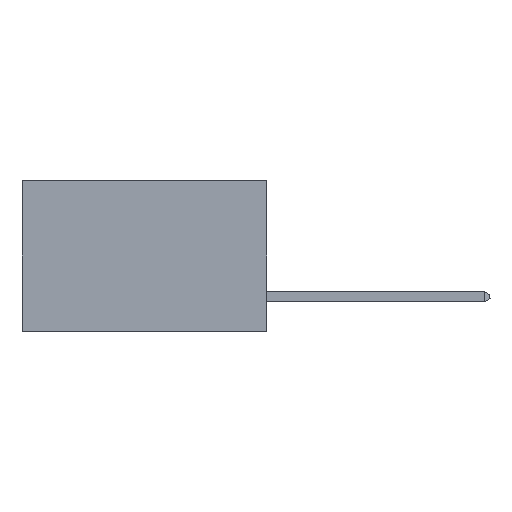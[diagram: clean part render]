
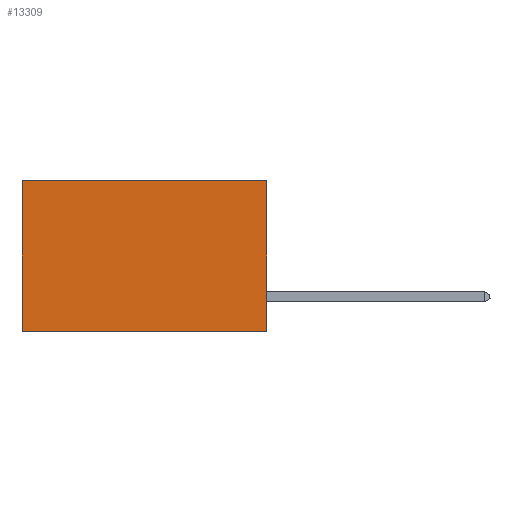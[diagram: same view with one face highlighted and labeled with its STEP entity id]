
A CAD part, left-side view. The second image highlights one B-rep face of the part: STEP entity #13309.
In plain terms, the highlighted planar face has unit normal (-1, 0, 0).
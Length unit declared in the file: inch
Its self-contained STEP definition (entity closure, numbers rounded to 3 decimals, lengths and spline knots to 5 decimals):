
#159 = AXIS2_PLACEMENT_3D ( 'NONE', #29523, #40713, #29852 ) ;
#1380 = ORIENTED_EDGE ( 'NONE', *, *, #31086, .F. ) ;
#3466 = PLANE ( 'NONE',  #159 ) ;
#7164 = EDGE_LOOP ( 'NONE', ( #7315, #12968, #1380, #22053 ) ) ;
#7315 = ORIENTED_EDGE ( 'NONE', *, *, #12239, .T. ) ;
#7946 = VERTEX_POINT ( 'NONE', #32042 ) ;
#8079 = CARTESIAN_POINT ( 'NONE',  ( 0.2875, 0.6, 0. ) ) ;
#8308 = CARTESIAN_POINT ( 'NONE',  ( 0.2875, 0., -0.37 ) ) ;
#10257 = EDGE_CURVE ( 'NONE', #40282, #7946, #44008, .T. ) ;
#11302 = CARTESIAN_POINT ( 'NONE',  ( 0.2875, 0., -0.37 ) ) ;
#11825 = DIRECTION ( 'NONE',  ( 0., 0., -1. ) ) ;
#12239 = EDGE_CURVE ( 'NONE', #7946, #24584, #40901, .T. ) ;
#12968 = ORIENTED_EDGE ( 'NONE', *, *, #41087, .F. ) ;
#13309 = ADVANCED_FACE ( 'NONE', ( #47727 ), #3466, .F. ) ;
#18860 = DIRECTION ( 'NONE',  ( 0., 0., -1. ) ) ;
#19154 = DIRECTION ( 'NONE',  ( 0., 1., 0. ) ) ;
#19657 = CARTESIAN_POINT ( 'NONE',  ( 0.2875, 0.6, -0.37 ) ) ;
#22053 = ORIENTED_EDGE ( 'NONE', *, *, #10257, .T. ) ;
#24584 = VERTEX_POINT ( 'NONE', #19657 ) ;
#26207 = DIRECTION ( 'NONE',  ( 0., 1., 0. ) ) ;
#26968 = VECTOR ( 'NONE', #19154, 39.37008 ) ;
#28718 = VECTOR ( 'NONE', #11825, 39.37008 ) ;
#28867 = VECTOR ( 'NONE', #18860, 39.37008 ) ;
#29321 = LINE ( 'NONE', #8308, #26968 ) ;
#29457 = CARTESIAN_POINT ( 'NONE',  ( 0.2875, 0., 0. ) ) ;
#29523 = CARTESIAN_POINT ( 'NONE',  ( 0.2875, 0., 0. ) ) ;
#29852 = DIRECTION ( 'NONE',  ( 0., 0., -1. ) ) ;
#30516 = CARTESIAN_POINT ( 'NONE',  ( 0.2875, 0., 0. ) ) ;
#31086 = EDGE_CURVE ( 'NONE', #40282, #38965, #35836, .T. ) ;
#32042 = CARTESIAN_POINT ( 'NONE',  ( 0.2875, 0.6, 0. ) ) ;
#33972 = CARTESIAN_POINT ( 'NONE',  ( 0.2875, 0., 0. ) ) ;
#34155 = VECTOR ( 'NONE', #26207, 39.37008 ) ;
#35836 = LINE ( 'NONE', #30516, #28867 ) ;
#38965 = VERTEX_POINT ( 'NONE', #11302 ) ;
#40282 = VERTEX_POINT ( 'NONE', #33972 ) ;
#40713 = DIRECTION ( 'NONE',  ( 1., 0., 0. ) ) ;
#40901 = LINE ( 'NONE', #8079, #28718 ) ;
#41087 = EDGE_CURVE ( 'NONE', #38965, #24584, #29321, .T. ) ;
#44008 = LINE ( 'NONE', #29457, #34155 ) ;
#47727 = FACE_OUTER_BOUND ( 'NONE', #7164, .T. ) ;
